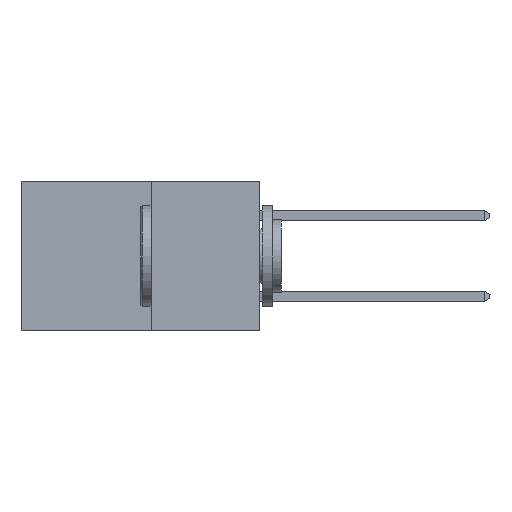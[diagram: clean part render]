
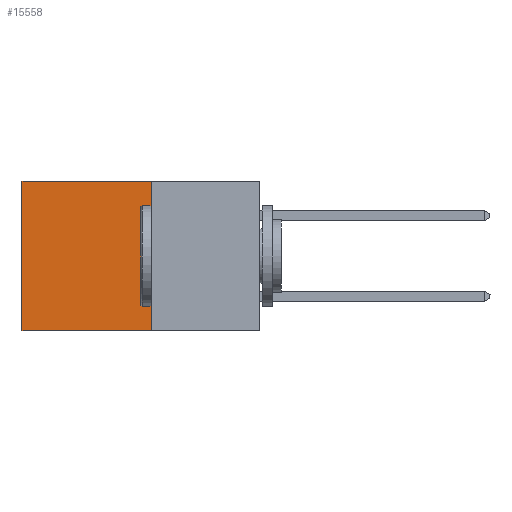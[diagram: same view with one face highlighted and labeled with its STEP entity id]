
A CAD part, left-side view. The second image highlights one B-rep face of the part: STEP entity #15558.
In plain terms, the highlighted planar face has unit normal (-1, 0, 0).
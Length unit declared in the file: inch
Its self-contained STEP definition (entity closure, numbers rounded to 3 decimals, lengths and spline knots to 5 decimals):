
#2008 = VECTOR ( 'NONE', #3460, 39.37008 ) ;
#2209 = FACE_OUTER_BOUND ( 'NONE', #14011, .T. ) ;
#2724 = VERTEX_POINT ( 'NONE', #28357 ) ;
#3460 = DIRECTION ( 'NONE',  ( 0., 1., 0. ) ) ;
#3739 = DIRECTION ( 'NONE',  ( 0., 0., -1. ) ) ;
#4390 = CARTESIAN_POINT ( 'NONE',  ( 0.277, 0.59, 0. ) ) ;
#6536 = LINE ( 'NONE', #23197, #18016 ) ;
#6703 = CARTESIAN_POINT ( 'NONE',  ( 0.277, 0.27, -0.37 ) ) ;
#7217 = ORIENTED_EDGE ( 'NONE', *, *, #24099, .T. ) ;
#7351 = CARTESIAN_POINT ( 'NONE',  ( 0.277, 0.27, -0.37 ) ) ;
#8267 = LINE ( 'NONE', #18916, #19729 ) ;
#9662 = DIRECTION ( 'NONE',  ( 1., 0., 0. ) ) ;
#9791 = DIRECTION ( 'NONE',  ( 0., 1., 0. ) ) ;
#11750 = DIRECTION ( 'NONE',  ( 0., 0., -1. ) ) ;
#11915 = ORIENTED_EDGE ( 'NONE', *, *, #29197, .T. ) ;
#11960 = LINE ( 'NONE', #19832, #18107 ) ;
#12421 = EDGE_CURVE ( 'NONE', #23083, #23845, #11960, .T. ) ;
#14011 = EDGE_LOOP ( 'NONE', ( #11915, #23211, #24260, #7217 ) ) ;
#14212 = LINE ( 'NONE', #26309, #2008 ) ;
#15558 = ADVANCED_FACE ( 'NONE', ( #2209 ), #21079, .F. ) ;
#16095 = VERTEX_POINT ( 'NONE', #4390 ) ;
#18016 = VECTOR ( 'NONE', #11750, 39.37008 ) ;
#18107 = VECTOR ( 'NONE', #3739, 39.37008 ) ;
#18916 = CARTESIAN_POINT ( 'NONE',  ( 0.277, 0.27, 0. ) ) ;
#19729 = VECTOR ( 'NONE', #9791, 39.37008 ) ;
#19832 = CARTESIAN_POINT ( 'NONE',  ( 0.277, 0.27, -0.37 ) ) ;
#20143 = CARTESIAN_POINT ( 'NONE',  ( 0.277, 0.27, 0. ) ) ;
#21079 = PLANE ( 'NONE',  #26883 ) ;
#23083 = VERTEX_POINT ( 'NONE', #20143 ) ;
#23197 = CARTESIAN_POINT ( 'NONE',  ( 0.277, 0.59, -0.37 ) ) ;
#23211 = ORIENTED_EDGE ( 'NONE', *, *, #25424, .F. ) ;
#23845 = VERTEX_POINT ( 'NONE', #6703 ) ;
#24099 = EDGE_CURVE ( 'NONE', #23083, #16095, #8267, .T. ) ;
#24260 = ORIENTED_EDGE ( 'NONE', *, *, #12421, .F. ) ;
#25424 = EDGE_CURVE ( 'NONE', #23845, #2724, #14212, .T. ) ;
#25650 = DIRECTION ( 'NONE',  ( 0., 0., -1. ) ) ;
#26309 = CARTESIAN_POINT ( 'NONE',  ( 0.277, 0.27, -0.37 ) ) ;
#26883 = AXIS2_PLACEMENT_3D ( 'NONE', #7351, #9662, #25650 ) ;
#28357 = CARTESIAN_POINT ( 'NONE',  ( 0.277, 0.59, -0.37 ) ) ;
#29197 = EDGE_CURVE ( 'NONE', #16095, #2724, #6536, .T. ) ;
